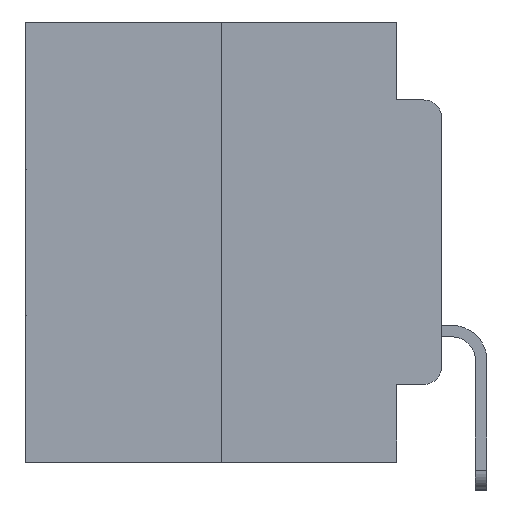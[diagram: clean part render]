
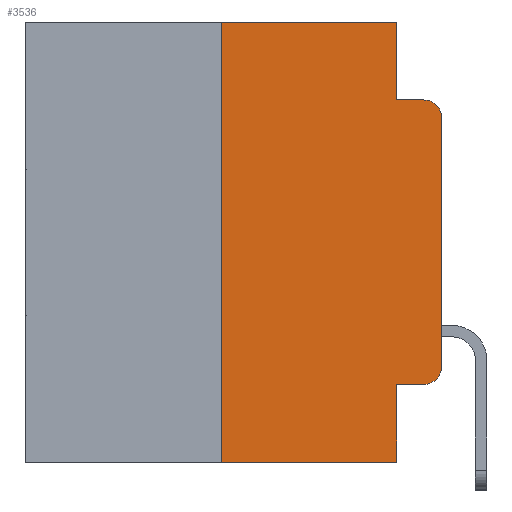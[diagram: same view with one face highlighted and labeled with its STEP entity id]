
A CAD part, left-side view. The second image highlights one B-rep face of the part: STEP entity #3536.
In plain terms, the highlighted planar face has unit normal (-1, 0, 0).
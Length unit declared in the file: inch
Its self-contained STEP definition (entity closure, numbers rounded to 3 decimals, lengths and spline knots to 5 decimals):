
#319 = EDGE_CURVE ( 'NONE', #25069, #11483, #23199, .T. ) ;
#332 = VECTOR ( 'NONE', #20925, 39.37008 ) ;
#489 = VERTEX_POINT ( 'NONE', #5192 ) ;
#1695 = LINE ( 'NONE', #2302, #332 ) ;
#1707 = DIRECTION ( 'NONE',  ( 0., -1., 0. ) ) ;
#1891 = DIRECTION ( 'NONE',  ( 0., -1., 0. ) ) ;
#2302 = CARTESIAN_POINT ( 'NONE',  ( 0., 0.473, 0. ) ) ;
#2588 = ORIENTED_EDGE ( 'NONE', *, *, #19568, .F. ) ;
#3049 = VECTOR ( 'NONE', #24776, 39.37008 ) ;
#3052 = VECTOR ( 'NONE', #25556, 39.37008 ) ;
#3536 = ADVANCED_FACE ( 'NONE', ( #17724 ), #5890, .F. ) ;
#4597 = CARTESIAN_POINT ( 'NONE',  ( 0., 0., -0.1085 ) ) ;
#4797 = ORIENTED_EDGE ( 'NONE', *, *, #7730, .T. ) ;
#4885 = LINE ( 'NONE', #13694, #25972 ) ;
#5019 = EDGE_CURVE ( 'NONE', #11483, #13611, #24655, .T. ) ;
#5192 = CARTESIAN_POINT ( 'NONE',  ( 0., 0.25, -0.5 ) ) ;
#5261 = VERTEX_POINT ( 'NONE', #4597 ) ;
#5643 = DIRECTION ( 'NONE',  ( 0., 0., -1. ) ) ;
#5699 = VERTEX_POINT ( 'NONE', #23951 ) ;
#5710 = LINE ( 'NONE', #6565, #3052 ) ;
#5890 = PLANE ( 'NONE',  #20251 ) ;
#6565 = CARTESIAN_POINT ( 'NONE',  ( 0., 0.051, -0.4115 ) ) ;
#7171 = EDGE_CURVE ( 'NONE', #489, #9662, #9708, .T. ) ;
#7649 = DIRECTION ( 'NONE',  ( -1., 0., 0. ) ) ;
#7725 = DIRECTION ( 'NONE',  ( 1., 0., 0. ) ) ;
#7730 = EDGE_CURVE ( 'NONE', #26937, #9242, #5710, .T. ) ;
#7872 = CARTESIAN_POINT ( 'NONE',  ( 0., 0.02, -0.0885 ) ) ;
#8632 = LINE ( 'NONE', #24437, #3049 ) ;
#9242 = VERTEX_POINT ( 'NONE', #20770 ) ;
#9546 = CARTESIAN_POINT ( 'NONE',  ( 0., 0.051, -0.4115 ) ) ;
#9662 = VERTEX_POINT ( 'NONE', #11545 ) ;
#9693 = CARTESIAN_POINT ( 'NONE',  ( 0., 0.02, -0.3915 ) ) ;
#9708 = LINE ( 'NONE', #24277, #15628 ) ;
#9965 = DIRECTION ( 'NONE',  ( 0., 0., -1. ) ) ;
#10413 = AXIS2_PLACEMENT_3D ( 'NONE', #9693, #7649, #22362 ) ;
#11483 = VERTEX_POINT ( 'NONE', #19792 ) ;
#11545 = CARTESIAN_POINT ( 'NONE',  ( 0., 0.051, -0.5 ) ) ;
#11767 = EDGE_CURVE ( 'NONE', #5261, #13611, #20924, .T. ) ;
#11820 = EDGE_CURVE ( 'NONE', #489, #21638, #8632, .T. ) ;
#12033 = AXIS2_PLACEMENT_3D ( 'NONE', #19249, #27323, #5643 ) ;
#13611 = VERTEX_POINT ( 'NONE', #7872 ) ;
#13647 = ORIENTED_EDGE ( 'NONE', *, *, #23115, .F. ) ;
#13694 = CARTESIAN_POINT ( 'NONE',  ( 0., 0.051, 0. ) ) ;
#13925 = CARTESIAN_POINT ( 'NONE',  ( 0., 0.25, 0. ) ) ;
#14629 = ORIENTED_EDGE ( 'NONE', *, *, #319, .F. ) ;
#14911 = VECTOR ( 'NONE', #19571, 39.37008 ) ;
#15233 = ORIENTED_EDGE ( 'NONE', *, *, #21640, .T. ) ;
#15304 = CARTESIAN_POINT ( 'NONE',  ( 0., 0.051, 0. ) ) ;
#15628 = VECTOR ( 'NONE', #1707, 39.37008 ) ;
#16472 = ORIENTED_EDGE ( 'NONE', *, *, #11820, .F. ) ;
#17359 = DIRECTION ( 'NONE',  ( 0., 0., 1. ) ) ;
#17614 = ORIENTED_EDGE ( 'NONE', *, *, #5019, .F. ) ;
#17724 = FACE_OUTER_BOUND ( 'NONE', #19536, .T. ) ;
#19249 = CARTESIAN_POINT ( 'NONE',  ( 0., 0.02, -0.1085 ) ) ;
#19536 = EDGE_LOOP ( 'NONE', ( #21756, #22031, #17614, #14629, #2588, #16472, #20732, #13647, #4797, #15233 ) ) ;
#19568 = EDGE_CURVE ( 'NONE', #21638, #25069, #1695, .T. ) ;
#19571 = DIRECTION ( 'NONE',  ( 0., 0., -1. ) ) ;
#19792 = CARTESIAN_POINT ( 'NONE',  ( 0., 0.051, -0.0885 ) ) ;
#20251 = AXIS2_PLACEMENT_3D ( 'NONE', #24893, #7725, #9965 ) ;
#20732 = ORIENTED_EDGE ( 'NONE', *, *, #7171, .T. ) ;
#20770 = CARTESIAN_POINT ( 'NONE',  ( 0., 0.02, -0.4115 ) ) ;
#20924 = CIRCLE ( 'NONE', #12033, 0.02 ) ;
#20925 = DIRECTION ( 'NONE',  ( 0., -1., 0. ) ) ;
#21514 = CARTESIAN_POINT ( 'NONE',  ( 0., 0., 0. ) ) ;
#21638 = VERTEX_POINT ( 'NONE', #13925 ) ;
#21640 = EDGE_CURVE ( 'NONE', #9242, #5699, #24654, .T. ) ;
#21679 = CARTESIAN_POINT ( 'NONE',  ( 0., 0.051, 0. ) ) ;
#21756 = ORIENTED_EDGE ( 'NONE', *, *, #26387, .T. ) ;
#22031 = ORIENTED_EDGE ( 'NONE', *, *, #11767, .T. ) ;
#22226 = DIRECTION ( 'NONE',  ( 0., 0., -1. ) ) ;
#22362 = DIRECTION ( 'NONE',  ( 0., 0., -1. ) ) ;
#23115 = EDGE_CURVE ( 'NONE', #26937, #9662, #4885, .T. ) ;
#23199 = LINE ( 'NONE', #15304, #14911 ) ;
#23951 = CARTESIAN_POINT ( 'NONE',  ( 0., 0., -0.3915 ) ) ;
#24152 = LINE ( 'NONE', #21514, #24487 ) ;
#24277 = CARTESIAN_POINT ( 'NONE',  ( 0., 0.473, -0.5 ) ) ;
#24437 = CARTESIAN_POINT ( 'NONE',  ( 0., 0.25, 0. ) ) ;
#24487 = VECTOR ( 'NONE', #17359, 39.37008 ) ;
#24654 = CIRCLE ( 'NONE', #10413, 0.02 ) ;
#24655 = LINE ( 'NONE', #25095, #25927 ) ;
#24776 = DIRECTION ( 'NONE',  ( 0., 0., 1. ) ) ;
#24893 = CARTESIAN_POINT ( 'NONE',  ( 0., 0.473, 0. ) ) ;
#25069 = VERTEX_POINT ( 'NONE', #21679 ) ;
#25095 = CARTESIAN_POINT ( 'NONE',  ( 0., 0.051, -0.0885 ) ) ;
#25556 = DIRECTION ( 'NONE',  ( 0., -1., 0. ) ) ;
#25927 = VECTOR ( 'NONE', #1891, 39.37008 ) ;
#25972 = VECTOR ( 'NONE', #22226, 39.37008 ) ;
#26387 = EDGE_CURVE ( 'NONE', #5699, #5261, #24152, .T. ) ;
#26937 = VERTEX_POINT ( 'NONE', #9546 ) ;
#27323 = DIRECTION ( 'NONE',  ( -1., 0., 0. ) ) ;
